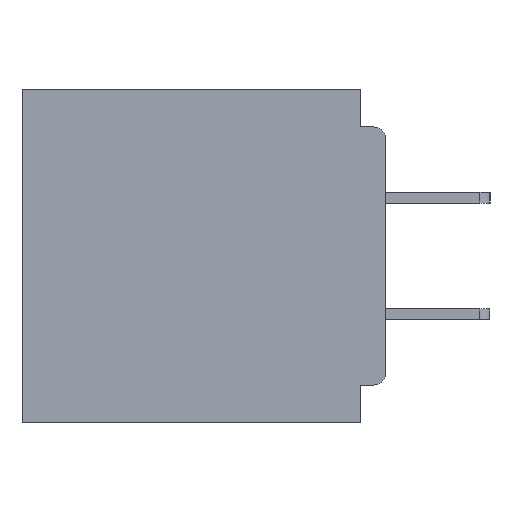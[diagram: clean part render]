
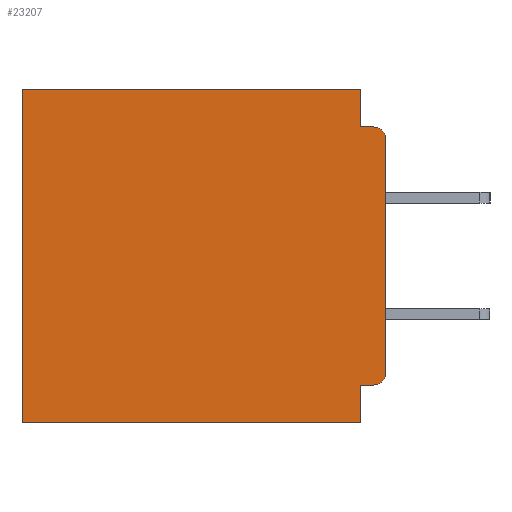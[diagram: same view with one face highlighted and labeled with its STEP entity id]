
A CAD part, left-side view. The second image highlights one B-rep face of the part: STEP entity #23207.
In plain terms, the highlighted planar face has unit normal (-1, 0, 0).
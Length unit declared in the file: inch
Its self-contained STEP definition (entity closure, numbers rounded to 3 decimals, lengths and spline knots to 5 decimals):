
#410 = VERTEX_POINT ( 'NONE', #19011 ) ;
#524 = DIRECTION ( 'NONE',  ( 0., 0., -1. ) ) ;
#795 = CARTESIAN_POINT ( 'NONE',  ( 0.3, 0.437, 0. ) ) ;
#1046 = CIRCLE ( 'NONE', #26327, 0.015 ) ;
#1442 = VERTEX_POINT ( 'NONE', #45092 ) ;
#1678 = EDGE_CURVE ( 'NONE', #56445, #4214, #1046, .T. ) ;
#2137 = VECTOR ( 'NONE', #54415, 39.37008 ) ;
#3528 = CARTESIAN_POINT ( 'NONE',  ( 0.3, 0., -0.045 ) ) ;
#3736 = CARTESIAN_POINT ( 'NONE',  ( 0.3, 0.437, -0.4 ) ) ;
#3745 = ORIENTED_EDGE ( 'NONE', *, *, #39741, .T. ) ;
#4214 = VERTEX_POINT ( 'NONE', #10756 ) ;
#8533 = DIRECTION ( 'NONE',  ( 0., 0., -1. ) ) ;
#8686 = AXIS2_PLACEMENT_3D ( 'NONE', #57229, #28857, #524 ) ;
#9390 = LINE ( 'NONE', #3528, #34547 ) ;
#9486 = CARTESIAN_POINT ( 'NONE',  ( 0.3, 0., 0. ) ) ;
#9658 = LINE ( 'NONE', #60525, #33306 ) ;
#10411 = CARTESIAN_POINT ( 'NONE',  ( 0.3, 0.437, -0.4 ) ) ;
#10756 = CARTESIAN_POINT ( 'NONE',  ( 0.3, 0., -0.34 ) ) ;
#11032 = LINE ( 'NONE', #9486, #45778 ) ;
#11274 = CARTESIAN_POINT ( 'NONE',  ( 0.3, 0.015, -0.355 ) ) ;
#11989 = AXIS2_PLACEMENT_3D ( 'NONE', #19146, #52296, #23889 ) ;
#17723 = EDGE_CURVE ( 'NONE', #1442, #410, #51148, .T. ) ;
#18332 = EDGE_CURVE ( 'NONE', #32978, #36416, #28089, .T. ) ;
#19011 = CARTESIAN_POINT ( 'NONE',  ( 0.3, 0.031, -0.045 ) ) ;
#19146 = CARTESIAN_POINT ( 'NONE',  ( 0.3, 0.015, -0.06 ) ) ;
#19743 = CARTESIAN_POINT ( 'NONE',  ( 0.3, 0., -0.06 ) ) ;
#20576 = CARTESIAN_POINT ( 'NONE',  ( 0.3, 0.031, -0.4 ) ) ;
#23207 = ADVANCED_FACE ( 'NONE', ( #31090 ), #42960, .F. ) ;
#23567 = ORIENTED_EDGE ( 'NONE', *, *, #42529, .F. ) ;
#23772 = VERTEX_POINT ( 'NONE', #19743 ) ;
#23889 = DIRECTION ( 'NONE',  ( 0., 0., -1. ) ) ;
#24207 = LINE ( 'NONE', #49724, #47925 ) ;
#26073 = ORIENTED_EDGE ( 'NONE', *, *, #17723, .F. ) ;
#26327 = AXIS2_PLACEMENT_3D ( 'NONE', #31045, #30980, #29597 ) ;
#26521 = ORIENTED_EDGE ( 'NONE', *, *, #37838, .F. ) ;
#27028 = DIRECTION ( 'NONE',  ( 0., 1., 0. ) ) ;
#27304 = LINE ( 'NONE', #49649, #2137 ) ;
#27438 = DIRECTION ( 'NONE',  ( 0., 0., -1. ) ) ;
#27509 = LINE ( 'NONE', #3736, #51231 ) ;
#28089 = LINE ( 'NONE', #50659, #39254 ) ;
#28857 = DIRECTION ( 'NONE',  ( 1., 0., 0. ) ) ;
#29197 = ORIENTED_EDGE ( 'NONE', *, *, #44155, .F. ) ;
#29367 = CARTESIAN_POINT ( 'NONE',  ( 0.3, 0.015, -0.045 ) ) ;
#29597 = DIRECTION ( 'NONE',  ( 0., 0., -1. ) ) ;
#30980 = DIRECTION ( 'NONE',  ( -1., 0., 0. ) ) ;
#31045 = CARTESIAN_POINT ( 'NONE',  ( 0.3, 0.015, -0.34 ) ) ;
#31090 = FACE_OUTER_BOUND ( 'NONE', #45791, .T. ) ;
#31837 = DIRECTION ( 'NONE',  ( 0., 0., -1. ) ) ;
#32978 = VERTEX_POINT ( 'NONE', #20576 ) ;
#33306 = VECTOR ( 'NONE', #27438, 39.37008 ) ;
#34235 = VERTEX_POINT ( 'NONE', #29367 ) ;
#34547 = VECTOR ( 'NONE', #36659, 39.37008 ) ;
#36416 = VERTEX_POINT ( 'NONE', #10411 ) ;
#36659 = DIRECTION ( 'NONE',  ( 0., -1., 0. ) ) ;
#37211 = ORIENTED_EDGE ( 'NONE', *, *, #44494, .T. ) ;
#37838 = EDGE_CURVE ( 'NONE', #56445, #54934, #24207, .T. ) ;
#38607 = VECTOR ( 'NONE', #31837, 39.37008 ) ;
#39254 = VECTOR ( 'NONE', #27028, 39.37008 ) ;
#39741 = EDGE_CURVE ( 'NONE', #23772, #34235, #57303, .T. ) ;
#41180 = ORIENTED_EDGE ( 'NONE', *, *, #1678, .T. ) ;
#42469 = CARTESIAN_POINT ( 'NONE',  ( 0.3, 0.031, -0.355 ) ) ;
#42529 = EDGE_CURVE ( 'NONE', #54934, #32978, #9658, .T. ) ;
#42960 = PLANE ( 'NONE',  #8686 ) ;
#44155 = EDGE_CURVE ( 'NONE', #23772, #4214, #27304, .T. ) ;
#44494 = EDGE_CURVE ( 'NONE', #1442, #61267, #11032, .T. ) ;
#45092 = CARTESIAN_POINT ( 'NONE',  ( 0.3, 0.031, 0. ) ) ;
#45778 = VECTOR ( 'NONE', #51910, 39.37008 ) ;
#45791 = EDGE_LOOP ( 'NONE', ( #29197, #3745, #50245, #26073, #37211, #55731, #50295, #23567, #26521, #41180 ) ) ;
#47925 = VECTOR ( 'NONE', #54496, 39.37008 ) ;
#49649 = CARTESIAN_POINT ( 'NONE',  ( 0.3, 0., -0.4 ) ) ;
#49724 = CARTESIAN_POINT ( 'NONE',  ( 0.3, 0., -0.355 ) ) ;
#50245 = ORIENTED_EDGE ( 'NONE', *, *, #54783, .F. ) ;
#50295 = ORIENTED_EDGE ( 'NONE', *, *, #18332, .F. ) ;
#50659 = CARTESIAN_POINT ( 'NONE',  ( 0.3, 0., -0.4 ) ) ;
#50721 = CARTESIAN_POINT ( 'NONE',  ( 0.3, 0.031, 0. ) ) ;
#51148 = LINE ( 'NONE', #50721, #38607 ) ;
#51231 = VECTOR ( 'NONE', #8533, 39.37008 ) ;
#51910 = DIRECTION ( 'NONE',  ( 0., 1., 0. ) ) ;
#52296 = DIRECTION ( 'NONE',  ( -1., 0., 0. ) ) ;
#54415 = DIRECTION ( 'NONE',  ( 0., 0., -1. ) ) ;
#54496 = DIRECTION ( 'NONE',  ( 0., 1., 0. ) ) ;
#54783 = EDGE_CURVE ( 'NONE', #410, #34235, #9390, .T. ) ;
#54934 = VERTEX_POINT ( 'NONE', #42469 ) ;
#55731 = ORIENTED_EDGE ( 'NONE', *, *, #56660, .T. ) ;
#56445 = VERTEX_POINT ( 'NONE', #11274 ) ;
#56660 = EDGE_CURVE ( 'NONE', #61267, #36416, #27509, .T. ) ;
#57229 = CARTESIAN_POINT ( 'NONE',  ( 0.3, 0., -0.4 ) ) ;
#57303 = CIRCLE ( 'NONE', #11989, 0.015 ) ;
#60525 = CARTESIAN_POINT ( 'NONE',  ( 0.3, 0.031, -0.4 ) ) ;
#61267 = VERTEX_POINT ( 'NONE', #795 ) ;
